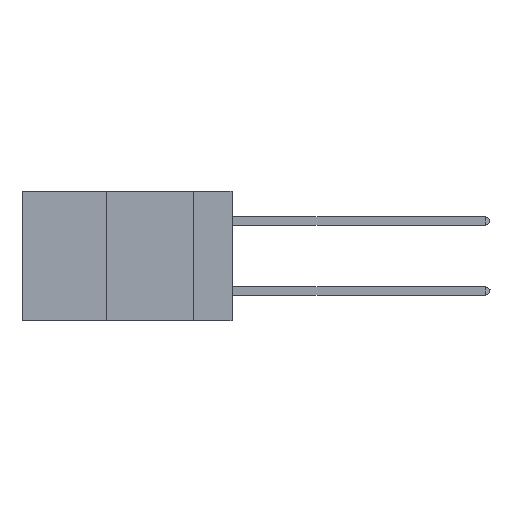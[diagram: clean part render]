
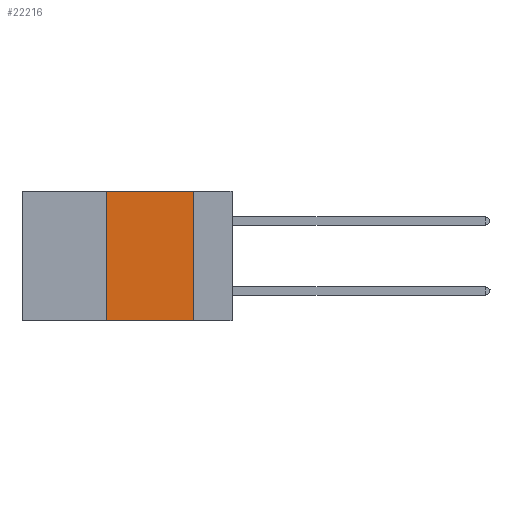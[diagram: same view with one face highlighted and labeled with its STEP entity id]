
A CAD part, left-side view. The second image highlights one B-rep face of the part: STEP entity #22216.
In plain terms, the highlighted planar face has unit normal (-1, 0, 0).
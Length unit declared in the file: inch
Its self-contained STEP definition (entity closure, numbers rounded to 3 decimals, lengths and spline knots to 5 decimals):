
#77 = ORIENTED_EDGE ( 'NONE', *, *, #14976, .F. ) ;
#614 = CARTESIAN_POINT ( 'NONE',  ( 0., 0.36, 0. ) ) ;
#1596 = ORIENTED_EDGE ( 'NONE', *, *, #4012, .T. ) ;
#2635 = DIRECTION ( 'NONE',  ( 0., -1., 0. ) ) ;
#4012 = EDGE_CURVE ( 'NONE', #19440, #26830, #6701, .T. ) ;
#4081 = CARTESIAN_POINT ( 'NONE',  ( 0., 0.36, 0. ) ) ;
#4958 = CARTESIAN_POINT ( 'NONE',  ( 0., 0.6, 0. ) ) ;
#6183 = VERTEX_POINT ( 'NONE', #614 ) ;
#6223 = DIRECTION ( 'NONE',  ( 1., 0., 0. ) ) ;
#6701 = LINE ( 'NONE', #25940, #17351 ) ;
#7151 = LINE ( 'NONE', #22732, #17961 ) ;
#8549 = DIRECTION ( 'NONE',  ( 0., 0., 1. ) ) ;
#8595 = PLANE ( 'NONE',  #26477 ) ;
#8795 = CARTESIAN_POINT ( 'NONE',  ( 0., 0.36, -0.37 ) ) ;
#9586 = VERTEX_POINT ( 'NONE', #23082 ) ;
#11007 = CARTESIAN_POINT ( 'NONE',  ( 0., 0.11, -0.37 ) ) ;
#14474 = CARTESIAN_POINT ( 'NONE',  ( 0., 0.6, 0. ) ) ;
#14976 = EDGE_CURVE ( 'NONE', #19440, #6183, #18938, .T. ) ;
#16999 = EDGE_CURVE ( 'NONE', #6183, #9586, #17585, .T. ) ;
#17351 = VECTOR ( 'NONE', #2635, 39.37008 ) ;
#17585 = LINE ( 'NONE', #4958, #26354 ) ;
#17961 = VECTOR ( 'NONE', #20206, 39.37008 ) ;
#18938 = LINE ( 'NONE', #4081, #25843 ) ;
#19440 = VERTEX_POINT ( 'NONE', #8795 ) ;
#19842 = DIRECTION ( 'NONE',  ( 0., -1., 0. ) ) ;
#20206 = DIRECTION ( 'NONE',  ( 0., 0., -1. ) ) ;
#20879 = ORIENTED_EDGE ( 'NONE', *, *, #16999, .F. ) ;
#20969 = FACE_OUTER_BOUND ( 'NONE', #25999, .T. ) ;
#22216 = ADVANCED_FACE ( 'NONE', ( #20969 ), #8595, .F. ) ;
#22732 = CARTESIAN_POINT ( 'NONE',  ( 0., 0.11, 0. ) ) ;
#22941 = EDGE_CURVE ( 'NONE', #9586, #26830, #7151, .T. ) ;
#23082 = CARTESIAN_POINT ( 'NONE',  ( 0., 0.11, 0. ) ) ;
#23356 = DIRECTION ( 'NONE',  ( 0., 0., -1. ) ) ;
#25843 = VECTOR ( 'NONE', #8549, 39.37008 ) ;
#25940 = CARTESIAN_POINT ( 'NONE',  ( 0., 0.6, -0.37 ) ) ;
#25999 = EDGE_LOOP ( 'NONE', ( #26594, #20879, #77, #1596 ) ) ;
#26354 = VECTOR ( 'NONE', #19842, 39.37008 ) ;
#26477 = AXIS2_PLACEMENT_3D ( 'NONE', #14474, #6223, #23356 ) ;
#26594 = ORIENTED_EDGE ( 'NONE', *, *, #22941, .F. ) ;
#26830 = VERTEX_POINT ( 'NONE', #11007 ) ;
